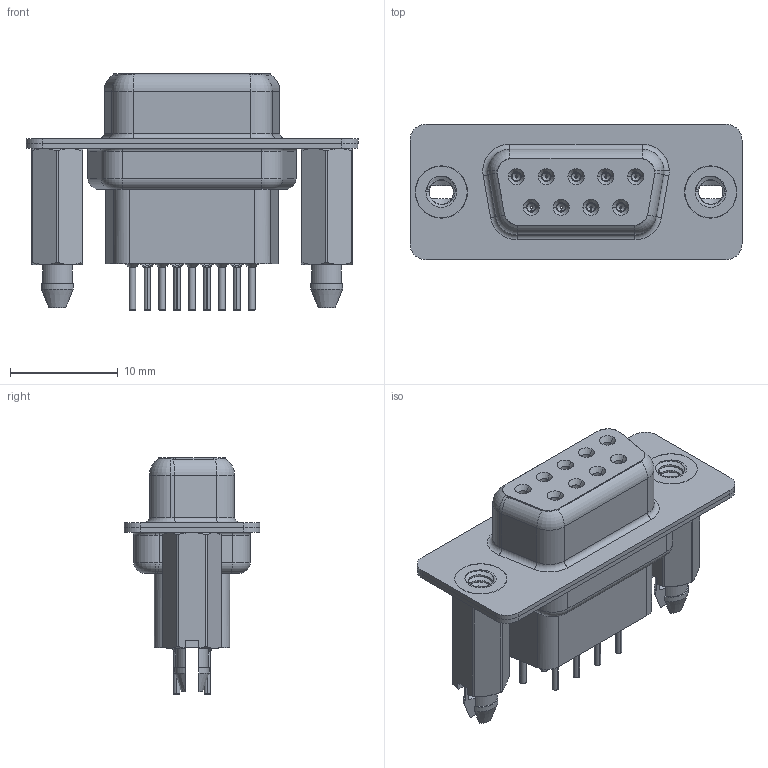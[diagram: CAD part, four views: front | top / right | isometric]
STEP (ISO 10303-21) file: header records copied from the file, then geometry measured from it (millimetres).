
FILE_DESCRIPTION (( 'STEP AP203' ), '1' );
FILE_NAME ('628-009-221-076.STEP', '2020-07-13T18:32:44', ( '' ), ( '' ), 'SwSTEP 2.0', 'SolidWorks 2020', '' );
FILE_SCHEMA (( 'CONFIG_CONTROL_DESIGN' ));
Length unit declared in the file: millimetre
Products named in the file (7): 628 Housing_09 HP; 628-009-221-076; 628 Shell Rear_09 Contacts; 628 Contact Row 2_21H; 628 Contact Row 1_21H; 628 Shell Front_09 Contacts; 628 4-40 Threaded Boardlock_HP
Assembly tree (14 placements, depth 2):
  628-009-221-076
    628 Housing_09 HP
    628 Shell Front_09 Contacts
    628 Shell Rear_09 Contacts
    628 Contact Row 1_21H  x5
    628 Contact Row 2_21H  x4
    628 4-40 Threaded Boardlock_HP  x2
Bounding box: 30.8 x 12.6 x 21.9 mm (x, y, z)
Volume: 2483.1 mm3; surface area: 5916.7 mm2
Topology: 14 solids, 14 shells, 1500 faces, 3881 edges, 2436 vertices
Faces by surface type: cylinder 502, plane 378, torus 279, bspline 190, cone 151
Entity records: 25184 total; most frequent: CARTESIAN_POINT 9217, ORIENTED_EDGE 3212, DIRECTION 3146, EDGE_CURVE 1606, AXIS2_PLACEMENT_3D 1285, VERTEX_POINT 1013, EDGE_LOOP 707, CIRCLE 673
